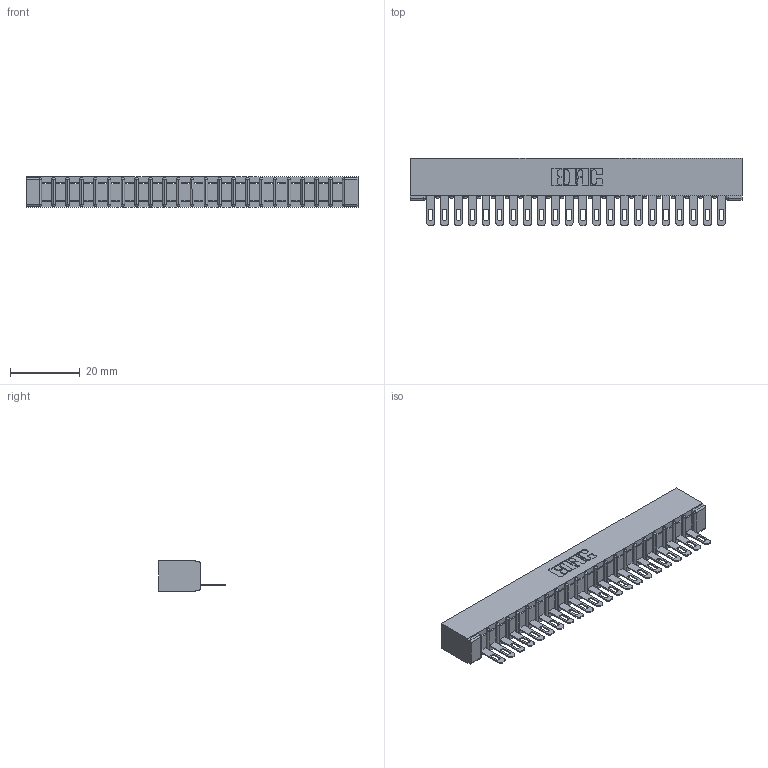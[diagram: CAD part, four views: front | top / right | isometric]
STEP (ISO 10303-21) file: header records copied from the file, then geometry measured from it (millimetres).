
FILE_DESCRIPTION (( 'STEP AP203' ), '1' );
FILE_NAME ('357-022-505-101.STEP', '2019-09-13T23:47:15', ( '' ), ( '' ), 'SwSTEP 2.0', 'SolidWorks 2016', '' );
FILE_SCHEMA (( 'CONFIG_CONTROL_DESIGN' ));
Length unit declared in the file: inch
Products named in the file (3): 357-022-505-101; 307-290-001_505; 307 Part_No Mounting Lugs
Assembly tree (23 placements, depth 2):
  357-022-505-101
    307 Part_No Mounting Lugs
    307-290-001_505  x22
Bounding box: 95.05 x 19.18 x 8.71 mm (x, y, z)
Volume: 6229.4 mm3; surface area: 10147.4 mm2
Topology: 23 solids, 23 shells, 1365 faces, 3863 edges, 2482 vertices
Faces by surface type: plane 858, cylinder 461, sphere 46
Entity records: 21022 total; most frequent: CARTESIAN_POINT 3532, ORIENTED_EDGE 3518, DIRECTION 3447, EDGE_CURVE 1759, LINE 1341, VECTOR 1341, VERTEX_POINT 1138, AXIS2_PLACEMENT_3D 1053
